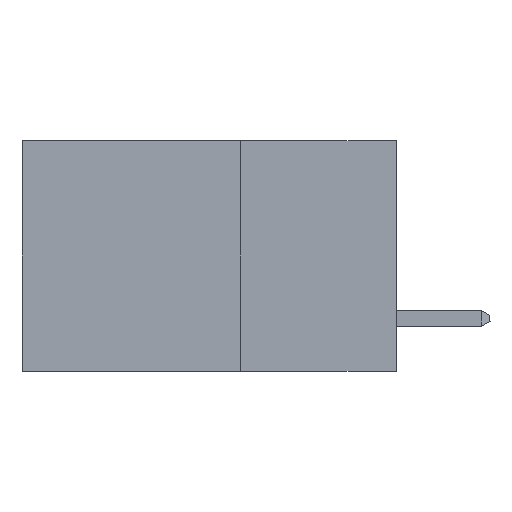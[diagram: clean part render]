
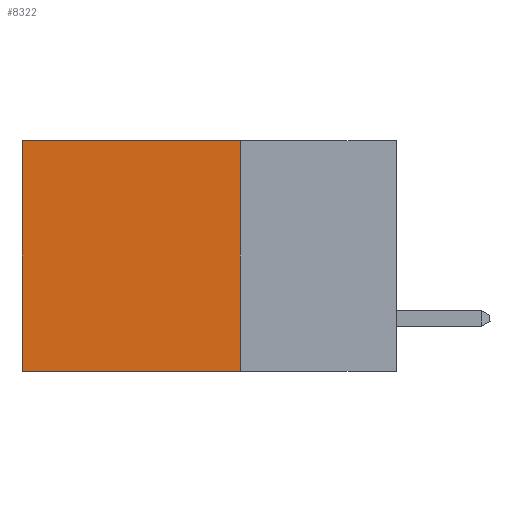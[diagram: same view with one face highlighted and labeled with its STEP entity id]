
A CAD part, left-side view. The second image highlights one B-rep face of the part: STEP entity #8322.
In plain terms, the highlighted planar face has unit normal (-1, 0, 0).
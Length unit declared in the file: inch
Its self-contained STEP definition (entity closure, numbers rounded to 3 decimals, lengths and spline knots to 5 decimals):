
#398 = CARTESIAN_POINT ( 'NONE',  ( 0.298, 0.25, 0. ) ) ;
#771 = VERTEX_POINT ( 'NONE', #3502 ) ;
#1712 = DIRECTION ( 'NONE',  ( 0., 0., -1. ) ) ;
#2100 = ORIENTED_EDGE ( 'NONE', *, *, #5574, .T. ) ;
#3044 = EDGE_CURVE ( 'NONE', #771, #13653, #4964, .T. ) ;
#3477 = LINE ( 'NONE', #9520, #6153 ) ;
#3502 = CARTESIAN_POINT ( 'NONE',  ( 0.298, 0.25, 0. ) ) ;
#3649 = VERTEX_POINT ( 'NONE', #11407 ) ;
#4414 = ORIENTED_EDGE ( 'NONE', *, *, #6913, .F. ) ;
#4650 = CARTESIAN_POINT ( 'NONE',  ( 0.298, 0.6, 0. ) ) ;
#4653 = VECTOR ( 'NONE', #13677, 39.37008 ) ;
#4853 = LINE ( 'NONE', #13517, #4653 ) ;
#4964 = LINE ( 'NONE', #398, #16527 ) ;
#5456 = CARTESIAN_POINT ( 'NONE',  ( 0.298, 0.6, -0.37 ) ) ;
#5574 = EDGE_CURVE ( 'NONE', #13653, #13950, #3477, .T. ) ;
#5684 = DIRECTION ( 'NONE',  ( 0., 0., -1. ) ) ;
#6153 = VECTOR ( 'NONE', #1712, 39.37008 ) ;
#6318 = EDGE_LOOP ( 'NONE', ( #2100, #4414, #17025, #14338 ) ) ;
#6913 = EDGE_CURVE ( 'NONE', #3649, #13950, #4853, .T. ) ;
#8322 = ADVANCED_FACE ( 'NONE', ( #13059 ), #12939, .F. ) ;
#8977 = CARTESIAN_POINT ( 'NONE',  ( 0.298, 0.25, 0. ) ) ;
#9257 = EDGE_CURVE ( 'NONE', #771, #3649, #12174, .T. ) ;
#9520 = CARTESIAN_POINT ( 'NONE',  ( 0.298, 0.6, 0. ) ) ;
#9907 = VECTOR ( 'NONE', #5684, 39.37008 ) ;
#10260 = DIRECTION ( 'NONE',  ( 1., 0., 0. ) ) ;
#10883 = DIRECTION ( 'NONE',  ( 0., 1., 0. ) ) ;
#11407 = CARTESIAN_POINT ( 'NONE',  ( 0.298, 0.25, -0.37 ) ) ;
#12174 = LINE ( 'NONE', #15142, #9907 ) ;
#12479 = AXIS2_PLACEMENT_3D ( 'NONE', #8977, #10260, #14302 ) ;
#12939 = PLANE ( 'NONE',  #12479 ) ;
#13059 = FACE_OUTER_BOUND ( 'NONE', #6318, .T. ) ;
#13517 = CARTESIAN_POINT ( 'NONE',  ( 0.298, 0.25, -0.37 ) ) ;
#13653 = VERTEX_POINT ( 'NONE', #4650 ) ;
#13677 = DIRECTION ( 'NONE',  ( 0., 1., 0. ) ) ;
#13950 = VERTEX_POINT ( 'NONE', #5456 ) ;
#14302 = DIRECTION ( 'NONE',  ( 0., 0., -1. ) ) ;
#14338 = ORIENTED_EDGE ( 'NONE', *, *, #3044, .T. ) ;
#15142 = CARTESIAN_POINT ( 'NONE',  ( 0.298, 0.25, 0. ) ) ;
#16527 = VECTOR ( 'NONE', #10883, 39.37008 ) ;
#17025 = ORIENTED_EDGE ( 'NONE', *, *, #9257, .F. ) ;
